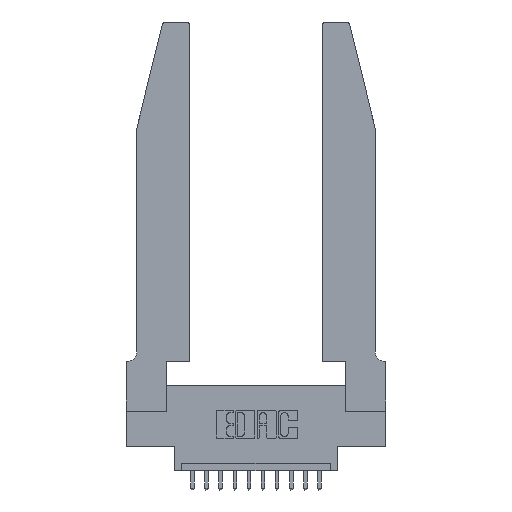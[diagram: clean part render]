
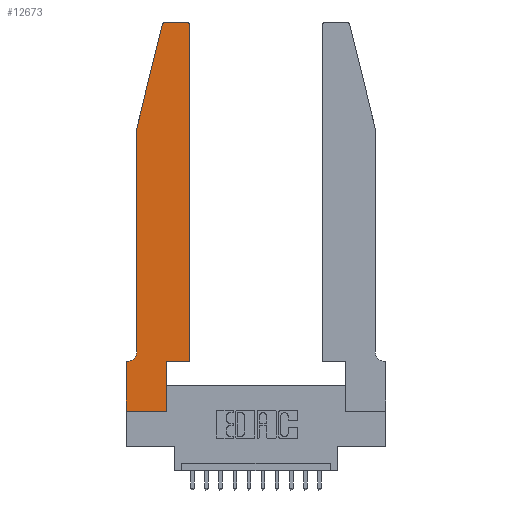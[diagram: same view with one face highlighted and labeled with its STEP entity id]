
A CAD part, top view. The second image highlights one B-rep face of the part: STEP entity #12673.
In plain terms, the highlighted planar face has unit normal (0, 0, 1).
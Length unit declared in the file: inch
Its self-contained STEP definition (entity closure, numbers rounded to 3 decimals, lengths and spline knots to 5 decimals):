
#55 = VERTEX_POINT ( 'NONE', #8275 ) ;
#148 = EDGE_CURVE ( 'NONE', #8894, #15426, #631, .T. ) ;
#244 = CARTESIAN_POINT ( 'NONE',  ( 0.0755, 0.42, 0.37 ) ) ;
#297 = EDGE_CURVE ( 'NONE', #15426, #9505, #5913, .T. ) ;
#631 = LINE ( 'NONE', #16520, #9080 ) ;
#984 = ORIENTED_EDGE ( 'NONE', *, *, #9672, .T. ) ;
#1621 = AXIS2_PLACEMENT_3D ( 'NONE', #6534, #15628, #2748 ) ;
#1925 = EDGE_CURVE ( 'NONE', #13077, #3638, #4235, .T. ) ;
#2044 = VECTOR ( 'NONE', #7851, 39.37008 ) ;
#2074 = VECTOR ( 'NONE', #9283, 39.37008 ) ;
#2177 = DIRECTION ( 'NONE',  ( 0., 0., 1. ) ) ;
#2225 = CARTESIAN_POINT ( 'NONE',  ( 0.25487, 2.72718, 0.37 ) ) ;
#2278 = LINE ( 'NONE', #4147, #2074 ) ;
#2402 = CARTESIAN_POINT ( 'NONE',  ( 0., 0., 0.37 ) ) ;
#2467 = VERTEX_POINT ( 'NONE', #7504 ) ;
#2748 = DIRECTION ( 'NONE',  ( 1., 0., 0. ) ) ;
#3199 = CARTESIAN_POINT ( 'NONE',  ( 0.4505, 0.35, 0.37 ) ) ;
#3260 = DIRECTION ( 'NONE',  ( 0., 1., 0. ) ) ;
#3416 = DIRECTION ( 'NONE',  ( 0., 0., 1. ) ) ;
#3499 = DIRECTION ( 'NONE',  ( 1., 0., 0. ) ) ;
#3546 = VERTEX_POINT ( 'NONE', #13955 ) ;
#3638 = VERTEX_POINT ( 'NONE', #4359 ) ;
#3736 = CIRCLE ( 'NONE', #10082, 0.03 ) ;
#3848 = CARTESIAN_POINT ( 'NONE',  ( 0.4505, 2.72, 0.37 ) ) ;
#3889 = ORIENTED_EDGE ( 'NONE', *, *, #11222, .T. ) ;
#3961 = CARTESIAN_POINT ( 'NONE',  ( 0.0755, 2., 0.37 ) ) ;
#4088 = LINE ( 'NONE', #15570, #14014 ) ;
#4147 = CARTESIAN_POINT ( 'NONE',  ( 0.0755, 0.35, 0.37 ) ) ;
#4159 = DIRECTION ( 'NONE',  ( 0., -1., 0. ) ) ;
#4235 = LINE ( 'NONE', #3961, #7415 ) ;
#4359 = CARTESIAN_POINT ( 'NONE',  ( 0.0755, 2., 0.37 ) ) ;
#4842 = AXIS2_PLACEMENT_3D ( 'NONE', #10561, #6721, #7789 ) ;
#4884 = EDGE_CURVE ( 'NONE', #2467, #10397, #11720, .T. ) ;
#4907 = ORIENTED_EDGE ( 'NONE', *, *, #13258, .T. ) ;
#5184 = CARTESIAN_POINT ( 'NONE',  ( 0., 0., 0.37 ) ) ;
#5272 = LINE ( 'NONE', #11541, #13354 ) ;
#5298 = CARTESIAN_POINT ( 'NONE',  ( 0., 0., 0.37 ) ) ;
#5778 = ORIENTED_EDGE ( 'NONE', *, *, #4884, .T. ) ;
#5913 = CIRCLE ( 'NONE', #1621, 0.03 ) ;
#6250 = ORIENTED_EDGE ( 'NONE', *, *, #297, .T. ) ;
#6458 = ORIENTED_EDGE ( 'NONE', *, *, #8777, .T. ) ;
#6534 = CARTESIAN_POINT ( 'NONE',  ( 0.4205, 2.72, 0.37 ) ) ;
#6721 = DIRECTION ( 'NONE',  ( 0., 0., -1. ) ) ;
#7415 = VECTOR ( 'NONE', #15319, 39.37008 ) ;
#7504 = CARTESIAN_POINT ( 'NONE',  ( 0., 0.35, 0.37 ) ) ;
#7605 = DIRECTION ( 'NONE',  ( 1., 0., 0. ) ) ;
#7789 = DIRECTION ( 'NONE',  ( -1., 0., 0. ) ) ;
#7851 = DIRECTION ( 'NONE',  ( 1., 0., 0. ) ) ;
#8004 = ORIENTED_EDGE ( 'NONE', *, *, #10745, .T. ) ;
#8275 = CARTESIAN_POINT ( 'NONE',  ( 0.0055, 0.35, 0.37 ) ) ;
#8477 = FACE_OUTER_BOUND ( 'NONE', #11368, .T. ) ;
#8777 = EDGE_CURVE ( 'NONE', #13181, #13077, #3736, .T. ) ;
#8894 = VERTEX_POINT ( 'NONE', #9008 ) ;
#8976 = VERTEX_POINT ( 'NONE', #14221 ) ;
#9008 = CARTESIAN_POINT ( 'NONE',  ( 0.4505, 0.35, 0.37 ) ) ;
#9062 = ORIENTED_EDGE ( 'NONE', *, *, #148, .T. ) ;
#9080 = VECTOR ( 'NONE', #11271, 39.37008 ) ;
#9113 = ORIENTED_EDGE ( 'NONE', *, *, #12449, .T. ) ;
#9283 = DIRECTION ( 'NONE',  ( -1., 0., 0. ) ) ;
#9458 = VECTOR ( 'NONE', #4159, 39.37008 ) ;
#9505 = VERTEX_POINT ( 'NONE', #9542 ) ;
#9542 = CARTESIAN_POINT ( 'NONE',  ( 0.4205, 2.75, 0.37 ) ) ;
#9672 = EDGE_CURVE ( 'NONE', #8976, #3546, #15433, .T. ) ;
#10060 = EDGE_CURVE ( 'NONE', #14304, #55, #13217, .T. ) ;
#10082 = AXIS2_PLACEMENT_3D ( 'NONE', #16620, #2177, #3499 ) ;
#10397 = VERTEX_POINT ( 'NONE', #2402 ) ;
#10561 = CARTESIAN_POINT ( 'NONE',  ( 0.0055, 0.42, 0.37 ) ) ;
#10745 = EDGE_CURVE ( 'NONE', #3546, #8894, #13049, .T. ) ;
#11033 = AXIS2_PLACEMENT_3D ( 'NONE', #11138, #3416, #7605 ) ;
#11138 = CARTESIAN_POINT ( 'NONE',  ( 0., 0.35, 0.37 ) ) ;
#11222 = EDGE_CURVE ( 'NONE', #55, #2467, #2278, .T. ) ;
#11247 = CARTESIAN_POINT ( 'NONE',  ( 0.2865, 0.35, 0.37 ) ) ;
#11271 = DIRECTION ( 'NONE',  ( 0., 1., 0. ) ) ;
#11368 = EDGE_LOOP ( 'NONE', ( #4907, #6458, #16273, #11975, #16411, #3889, #5778, #9113, #984, #8004, #9062, #6250 ) ) ;
#11541 = CARTESIAN_POINT ( 'NONE',  ( 0.2605, 2.75, 0.37 ) ) ;
#11596 = VECTOR ( 'NONE', #3260, 39.37008 ) ;
#11720 = LINE ( 'NONE', #5298, #9458 ) ;
#11975 = ORIENTED_EDGE ( 'NONE', *, *, #12401, .T. ) ;
#12401 = EDGE_CURVE ( 'NONE', #3638, #14304, #4088, .T. ) ;
#12449 = EDGE_CURVE ( 'NONE', #10397, #8976, #15806, .T. ) ;
#12673 = ADVANCED_FACE ( 'NONE', ( #8477 ), #14169, .T. ) ;
#12847 = DIRECTION ( 'NONE',  ( -1., 0., 0. ) ) ;
#13049 = LINE ( 'NONE', #3199, #14667 ) ;
#13077 = VERTEX_POINT ( 'NONE', #2225 ) ;
#13181 = VERTEX_POINT ( 'NONE', #16310 ) ;
#13217 = CIRCLE ( 'NONE', #4842, 0.07 ) ;
#13258 = EDGE_CURVE ( 'NONE', #9505, #13181, #5272, .T. ) ;
#13354 = VECTOR ( 'NONE', #12847, 39.37008 ) ;
#13955 = CARTESIAN_POINT ( 'NONE',  ( 0.2865, 0.35, 0.37 ) ) ;
#14014 = VECTOR ( 'NONE', #15674, 39.37008 ) ;
#14169 = PLANE ( 'NONE',  #11033 ) ;
#14221 = CARTESIAN_POINT ( 'NONE',  ( 0.2865, 0., 0.37 ) ) ;
#14304 = VERTEX_POINT ( 'NONE', #244 ) ;
#14667 = VECTOR ( 'NONE', #15021, 39.37008 ) ;
#15021 = DIRECTION ( 'NONE',  ( 1., 0., 0. ) ) ;
#15319 = DIRECTION ( 'NONE',  ( -0.239, -0.971, 0. ) ) ;
#15426 = VERTEX_POINT ( 'NONE', #3848 ) ;
#15433 = LINE ( 'NONE', #11247, #11596 ) ;
#15570 = CARTESIAN_POINT ( 'NONE',  ( 0.0755, 2., 0.37 ) ) ;
#15628 = DIRECTION ( 'NONE',  ( 0., 0., 1. ) ) ;
#15674 = DIRECTION ( 'NONE',  ( 0., -1., 0. ) ) ;
#15806 = LINE ( 'NONE', #5184, #2044 ) ;
#16273 = ORIENTED_EDGE ( 'NONE', *, *, #1925, .T. ) ;
#16310 = CARTESIAN_POINT ( 'NONE',  ( 0.284, 2.75, 0.37 ) ) ;
#16411 = ORIENTED_EDGE ( 'NONE', *, *, #10060, .T. ) ;
#16520 = CARTESIAN_POINT ( 'NONE',  ( 0.4505, 0.35, 0.37 ) ) ;
#16620 = CARTESIAN_POINT ( 'NONE',  ( 0.284, 2.72, 0.37 ) ) ;
